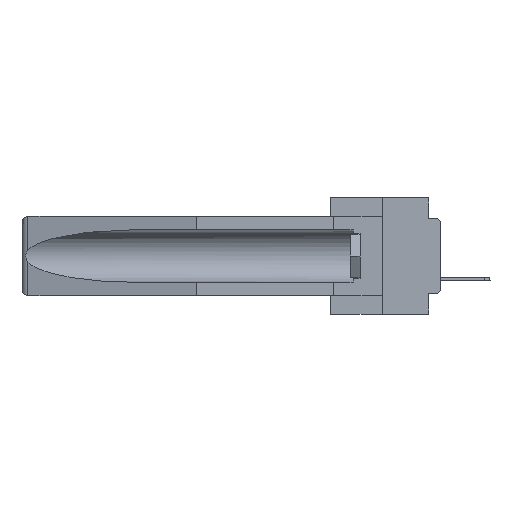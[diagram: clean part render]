
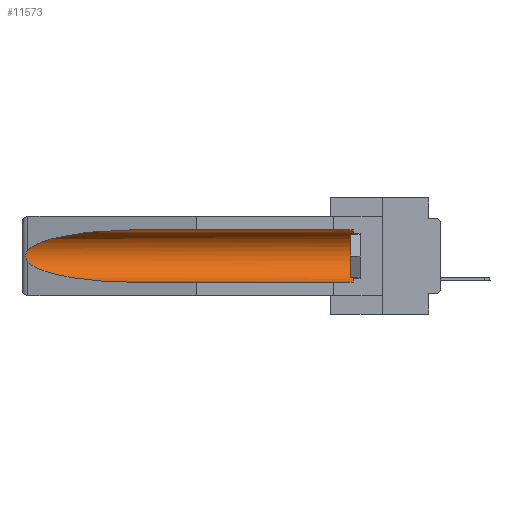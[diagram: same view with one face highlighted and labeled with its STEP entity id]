
A CAD part, left-side view. The second image highlights one B-rep face of the part: STEP entity #11573.
In plain terms, the highlighted cylindrical face has radius 2.857 mm (diameter 5.715 mm), a partial arc.
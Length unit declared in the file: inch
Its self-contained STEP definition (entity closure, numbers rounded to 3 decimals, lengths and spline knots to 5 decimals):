
#525 = CARTESIAN_POINT ( 'NONE',  ( 0.26537, 1.52718, -0.14972 ) ) ;
#703 = CARTESIAN_POINT ( 'NONE',  ( 0.26655, 1.53094, -0.18657 ) ) ;
#1178 = DIRECTION ( 'NONE',  ( 0., -1., 0. ) ) ;
#1193 = VECTOR ( 'NONE', #13803, 39.37008 ) ;
#1346 = CARTESIAN_POINT ( 'NONE',  ( 0.155, 0.126, -0.284 ) ) ;
#1548 = EDGE_LOOP ( 'NONE', ( #24899, #34813, #30332, #27445, #36183, #17673 ) ) ;
#2633 = CARTESIAN_POINT ( 'NONE',  ( 0.155, -0.30754, -0.284 ) ) ;
#2658 = AXIS2_PLACEMENT_3D ( 'NONE', #35602, #7940, #19100 ) ;
#2995 = CARTESIAN_POINT ( 'NONE',  ( 0.25451, 1.48313, -0.24835 ) ) ;
#3913 = VECTOR ( 'NONE', #13282, 39.37008 ) ;
#4078 = CARTESIAN_POINT ( 'NONE',  ( 0.155, 1.07973, -0.059 ) ) ;
#7940 = DIRECTION ( 'NONE',  ( 0., 1., 0. ) ) ;
#8070 =( BOUNDED_CURVE ( )  B_SPLINE_CURVE ( 3, ( #11278, #33451, #27942, #11106 ),
 .UNSPECIFIED., .F., .F. ) 
 B_SPLINE_CURVE_WITH_KNOTS ( ( 4, 4 ),
 ( 4.71239, 6.08839 ),
 .UNSPECIFIED. ) 
 CURVE ( )  GEOMETRIC_REPRESENTATION_ITEM ( )  RATIONAL_B_SPLINE_CURVE ( ( 1., 0.848, 0.848, 1. ) ) 
 REPRESENTATION_ITEM ( '' )  );
#9171 = CARTESIAN_POINT ( 'NONE',  ( 0.26597, 1.5296, -0.19026 ) ) ;
#9628 = CARTESIAN_POINT ( 'NONE',  ( 0.155, 0.126, -0.1715 ) ) ;
#9880 = CARTESIAN_POINT ( 'NONE',  ( 0.2673, 1.53269, -0.17917 ) ) ;
#11106 = CARTESIAN_POINT ( 'NONE',  ( 0.26537, 1.52718, -0.14972 ) ) ;
#11278 = CARTESIAN_POINT ( 'NONE',  ( 0.155, 1.07973, -0.059 ) ) ;
#11573 = ADVANCED_FACE ( 'NONE', ( #21304 ), #35234, .F. ) ;
#11716 = CARTESIAN_POINT ( 'NONE',  ( 0.26597, 1.52961, -0.15275 ) ) ;
#13282 = DIRECTION ( 'NONE',  ( 0., 1., 0. ) ) ;
#13446 = EDGE_CURVE ( 'NONE', #36158, #16096, #33150, .T. ) ;
#13803 = DIRECTION ( 'NONE',  ( 0., 1., 0. ) ) ;
#13809 = EDGE_CURVE ( 'NONE', #28958, #36158, #8070, .T. ) ;
#13942 = EDGE_CURVE ( 'NONE', #24150, #24847, #31119, .T. ) ;
#14367 =( BOUNDED_CURVE ( )  B_SPLINE_CURVE ( 3, ( #28089, #2995, #19314, #25338 ),
 .UNSPECIFIED., .F., .F. ) 
 B_SPLINE_CURVE_WITH_KNOTS ( ( 4, 4 ),
 ( 0.1948, 1.5708 ),
 .UNSPECIFIED. ) 
 CURVE ( )  GEOMETRIC_REPRESENTATION_ITEM ( )  RATIONAL_B_SPLINE_CURVE ( ( 1., 0.848, 0.848, 1. ) ) 
 REPRESENTATION_ITEM ( '' )  );
#15326 = AXIS2_PLACEMENT_3D ( 'NONE', #9628, #1178, #26099 ) ;
#16096 = VERTEX_POINT ( 'NONE', #26870 ) ;
#16697 = CARTESIAN_POINT ( 'NONE',  ( 0.26537, 1.52718, -0.14972 ) ) ;
#17673 = ORIENTED_EDGE ( 'NONE', *, *, #35661, .T. ) ;
#17795 = CARTESIAN_POINT ( 'NONE',  ( 0.155, 1.07973, -0.284 ) ) ;
#18127 = CARTESIAN_POINT ( 'NONE',  ( 0.26537, 1.52718, -0.19328 ) ) ;
#19100 = DIRECTION ( 'NONE',  ( 0., 0., 1. ) ) ;
#19314 = CARTESIAN_POINT ( 'NONE',  ( 0.21114, 1.30732, -0.284 ) ) ;
#21304 = FACE_OUTER_BOUND ( 'NONE', #1548, .T. ) ;
#21858 = LINE ( 'NONE', #22394, #1193 ) ;
#22394 = CARTESIAN_POINT ( 'NONE',  ( 0.155, -0.30754, -0.059 ) ) ;
#22877 = CARTESIAN_POINT ( 'NONE',  ( 0.26654, 1.53092, -0.15636 ) ) ;
#23065 = CARTESIAN_POINT ( 'NONE',  ( 0.2675, 1.53308, -0.17534 ) ) ;
#24150 = VERTEX_POINT ( 'NONE', #1346 ) ;
#24847 = VERTEX_POINT ( 'NONE', #30596 ) ;
#24899 = ORIENTED_EDGE ( 'NONE', *, *, #13809, .T. ) ;
#25338 = CARTESIAN_POINT ( 'NONE',  ( 0.155, 1.07973, -0.284 ) ) ;
#26099 = DIRECTION ( 'NONE',  ( 0., 0., 1. ) ) ;
#26870 = CARTESIAN_POINT ( 'NONE',  ( 0.26537, 1.52718, -0.19328 ) ) ;
#27445 = ORIENTED_EDGE ( 'NONE', *, *, #30309, .F. ) ;
#27728 = LINE ( 'NONE', #2633, #3913 ) ;
#27942 = CARTESIAN_POINT ( 'NONE',  ( 0.25451, 1.48313, -0.09465 ) ) ;
#28089 = CARTESIAN_POINT ( 'NONE',  ( 0.26537, 1.52718, -0.19328 ) ) ;
#28958 = VERTEX_POINT ( 'NONE', #4078 ) ;
#30309 = EDGE_CURVE ( 'NONE', #24150, #30715, #27728, .T. ) ;
#30332 = ORIENTED_EDGE ( 'NONE', *, *, #31227, .T. ) ;
#30596 = CARTESIAN_POINT ( 'NONE',  ( 0.155, 0.126, -0.059 ) ) ;
#30715 = VERTEX_POINT ( 'NONE', #17795 ) ;
#31119 = CIRCLE ( 'NONE', #15326, 0.1125 ) ;
#31227 = EDGE_CURVE ( 'NONE', #16096, #30715, #14367, .T. ) ;
#33150 = B_SPLINE_CURVE_WITH_KNOTS ( 'NONE', 3,
 ( #525, #11716, #22877, #34058, #36107, #23065, #9880, #703, #9171, #18127 ),
 .UNSPECIFIED., .F., .F.,
 ( 4, 2, 2, 2, 4 ),
 ( 0., 0.00029, 0.00058, 0.00087, 0.00117 ),
 .UNSPECIFIED. ) ;
#33451 = CARTESIAN_POINT ( 'NONE',  ( 0.21114, 1.30732, -0.059 ) ) ;
#34058 = CARTESIAN_POINT ( 'NONE',  ( 0.2673, 1.5327, -0.16383 ) ) ;
#34813 = ORIENTED_EDGE ( 'NONE', *, *, #13446, .T. ) ;
#35234 = CYLINDRICAL_SURFACE ( 'NONE', #2658, 0.1125 ) ;
#35602 = CARTESIAN_POINT ( 'NONE',  ( 0.155, -0.30754, -0.1715 ) ) ;
#35661 = EDGE_CURVE ( 'NONE', #24847, #28958, #21858, .T. ) ;
#36107 = CARTESIAN_POINT ( 'NONE',  ( 0.2675, 1.53308, -0.16763 ) ) ;
#36158 = VERTEX_POINT ( 'NONE', #16697 ) ;
#36183 = ORIENTED_EDGE ( 'NONE', *, *, #13942, .T. ) ;
